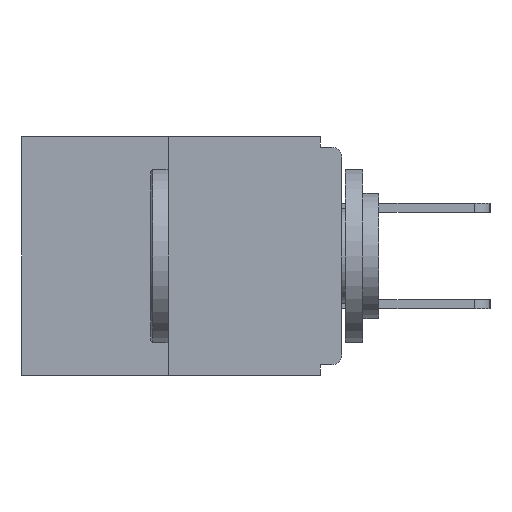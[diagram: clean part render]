
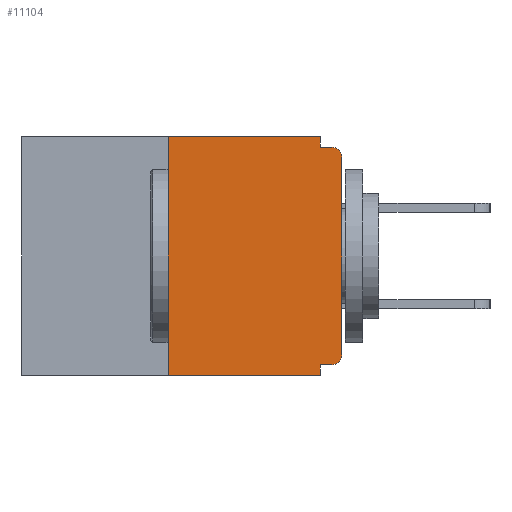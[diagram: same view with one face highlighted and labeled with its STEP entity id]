
A CAD part, left-side view. The second image highlights one B-rep face of the part: STEP entity #11104.
In plain terms, the highlighted planar face has unit normal (-1, 0, 0).
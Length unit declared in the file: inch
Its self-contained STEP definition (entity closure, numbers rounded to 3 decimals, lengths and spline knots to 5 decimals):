
#8 = EDGE_CURVE ( 'NONE', #4992, #4539, #4705, .T. ) ;
#120 = VERTEX_POINT ( 'NONE', #2531 ) ;
#148 = CARTESIAN_POINT ( 'NONE',  ( 0., 0., -0.015 ) ) ;
#259 = EDGE_CURVE ( 'NONE', #13724, #120, #8931, .T. ) ;
#627 = DIRECTION ( 'NONE',  ( 0., -1., 0. ) ) ;
#884 = CARTESIAN_POINT ( 'NONE',  ( 0., 0.015, -0.328 ) ) ;
#920 = DIRECTION ( 'NONE',  ( -1., 0., 0. ) ) ;
#985 = ORIENTED_EDGE ( 'NONE', *, *, #13694, .T. ) ;
#1216 = DIRECTION ( 'NONE',  ( 0., 0., -1. ) ) ;
#1575 = CARTESIAN_POINT ( 'NONE',  ( 0., 0., -0.328 ) ) ;
#1670 = AXIS2_PLACEMENT_3D ( 'NONE', #9193, #15257, #15044 ) ;
#1727 = VECTOR ( 'NONE', #11707, 39.37008 ) ;
#1987 = DIRECTION ( 'NONE',  ( 0., 0., -1. ) ) ;
#2192 = AXIS2_PLACEMENT_3D ( 'NONE', #8605, #6129, #1216 ) ;
#2514 = EDGE_CURVE ( 'NONE', #13350, #13724, #13576, .T. ) ;
#2531 = CARTESIAN_POINT ( 'NONE',  ( 0., 0.031, -0.015 ) ) ;
#3064 = DIRECTION ( 'NONE',  ( 0., -1., 0. ) ) ;
#3222 = ORIENTED_EDGE ( 'NONE', *, *, #4940, .F. ) ;
#3493 = EDGE_CURVE ( 'NONE', #9925, #9335, #15425, .T. ) ;
#3513 = VECTOR ( 'NONE', #3064, 39.37008 ) ;
#3562 = ORIENTED_EDGE ( 'NONE', *, *, #259, .F. ) ;
#3852 = DIRECTION ( 'NONE',  ( 0., 0., -1. ) ) ;
#3958 = VERTEX_POINT ( 'NONE', #15155 ) ;
#4289 = LINE ( 'NONE', #148, #5634 ) ;
#4325 = VECTOR ( 'NONE', #1987, 39.37008 ) ;
#4442 = LINE ( 'NONE', #15541, #9830 ) ;
#4539 = VERTEX_POINT ( 'NONE', #10983 ) ;
#4705 = CIRCLE ( 'NONE', #7262, 0.015 ) ;
#4802 = EDGE_CURVE ( 'NONE', #4918, #9335, #10017, .T. ) ;
#4825 = ORIENTED_EDGE ( 'NONE', *, *, #8, .T. ) ;
#4918 = VERTEX_POINT ( 'NONE', #7208 ) ;
#4940 = EDGE_CURVE ( 'NONE', #4918, #13350, #4442, .T. ) ;
#4978 = CARTESIAN_POINT ( 'NONE',  ( 0., 0.031, -0.343 ) ) ;
#4992 = VERTEX_POINT ( 'NONE', #8872 ) ;
#5125 = CARTESIAN_POINT ( 'NONE',  ( 0., 0.46, 0. ) ) ;
#5500 = PLANE ( 'NONE',  #1670 ) ;
#5634 = VECTOR ( 'NONE', #12355, 39.37008 ) ;
#5862 = LINE ( 'NONE', #15451, #15526 ) ;
#5982 = DIRECTION ( 'NONE',  ( 0., 0., 1. ) ) ;
#6129 = DIRECTION ( 'NONE',  ( -1., 0., 0. ) ) ;
#7208 = CARTESIAN_POINT ( 'NONE',  ( 0., 0.25, -0.343 ) ) ;
#7262 = AXIS2_PLACEMENT_3D ( 'NONE', #9542, #920, #10654 ) ;
#7653 = FACE_OUTER_BOUND ( 'NONE', #9748, .T. ) ;
#8605 = CARTESIAN_POINT ( 'NONE',  ( 0., 0.015, -0.313 ) ) ;
#8872 = CARTESIAN_POINT ( 'NONE',  ( 0., 0., -0.03 ) ) ;
#8931 = LINE ( 'NONE', #9020, #4325 ) ;
#9020 = CARTESIAN_POINT ( 'NONE',  ( 0., 0.031, 0. ) ) ;
#9193 = CARTESIAN_POINT ( 'NONE',  ( 0., 0.46, 0. ) ) ;
#9220 = ORIENTED_EDGE ( 'NONE', *, *, #9526, .F. ) ;
#9334 = CARTESIAN_POINT ( 'NONE',  ( 0., 0.031, -0.343 ) ) ;
#9335 = VERTEX_POINT ( 'NONE', #9334 ) ;
#9526 = EDGE_CURVE ( 'NONE', #120, #4539, #4289, .T. ) ;
#9542 = CARTESIAN_POINT ( 'NONE',  ( 0., 0.015, -0.03 ) ) ;
#9634 = VECTOR ( 'NONE', #627, 39.37008 ) ;
#9748 = EDGE_LOOP ( 'NONE', ( #15620, #3222, #11259, #14486, #13102, #11661, #985, #4825, #9220, #3562 ) ) ;
#9830 = VECTOR ( 'NONE', #5982, 39.37008 ) ;
#9925 = VERTEX_POINT ( 'NONE', #13321 ) ;
#10017 = LINE ( 'NONE', #15062, #3513 ) ;
#10339 = VECTOR ( 'NONE', #3852, 39.37008 ) ;
#10654 = DIRECTION ( 'NONE',  ( 0., 0., -1. ) ) ;
#10673 = DIRECTION ( 'NONE',  ( 0., 0., 1. ) ) ;
#10983 = CARTESIAN_POINT ( 'NONE',  ( 0., 0.015, -0.015 ) ) ;
#11104 = ADVANCED_FACE ( 'NONE', ( #7653 ), #5500, .F. ) ;
#11259 = ORIENTED_EDGE ( 'NONE', *, *, #4802, .T. ) ;
#11661 = ORIENTED_EDGE ( 'NONE', *, *, #12625, .T. ) ;
#11707 = DIRECTION ( 'NONE',  ( 0., 1., 0. ) ) ;
#12355 = DIRECTION ( 'NONE',  ( 0., -1., 0. ) ) ;
#12482 = EDGE_CURVE ( 'NONE', #15302, #9925, #14055, .T. ) ;
#12625 = EDGE_CURVE ( 'NONE', #15302, #3958, #13127, .T. ) ;
#12980 = CARTESIAN_POINT ( 'NONE',  ( 0., 0.25, 0. ) ) ;
#13102 = ORIENTED_EDGE ( 'NONE', *, *, #12482, .F. ) ;
#13127 = CIRCLE ( 'NONE', #2192, 0.015 ) ;
#13321 = CARTESIAN_POINT ( 'NONE',  ( 0., 0.031, -0.328 ) ) ;
#13350 = VERTEX_POINT ( 'NONE', #12980 ) ;
#13576 = LINE ( 'NONE', #5125, #9634 ) ;
#13653 = CARTESIAN_POINT ( 'NONE',  ( 0., 0.031, 0. ) ) ;
#13694 = EDGE_CURVE ( 'NONE', #3958, #4992, #5862, .T. ) ;
#13724 = VERTEX_POINT ( 'NONE', #13653 ) ;
#14055 = LINE ( 'NONE', #1575, #1727 ) ;
#14486 = ORIENTED_EDGE ( 'NONE', *, *, #3493, .F. ) ;
#15044 = DIRECTION ( 'NONE',  ( 0., 0., -1. ) ) ;
#15062 = CARTESIAN_POINT ( 'NONE',  ( 0., 0.46, -0.343 ) ) ;
#15155 = CARTESIAN_POINT ( 'NONE',  ( 0., 0., -0.313 ) ) ;
#15257 = DIRECTION ( 'NONE',  ( 1., 0., 0. ) ) ;
#15302 = VERTEX_POINT ( 'NONE', #884 ) ;
#15425 = LINE ( 'NONE', #4978, #10339 ) ;
#15451 = CARTESIAN_POINT ( 'NONE',  ( 0., 0., 0. ) ) ;
#15526 = VECTOR ( 'NONE', #10673, 39.37008 ) ;
#15541 = CARTESIAN_POINT ( 'NONE',  ( 0., 0.25, 0. ) ) ;
#15620 = ORIENTED_EDGE ( 'NONE', *, *, #2514, .F. ) ;
